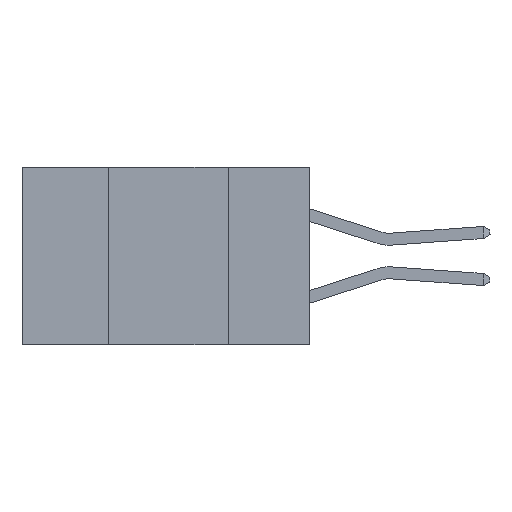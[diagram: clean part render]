
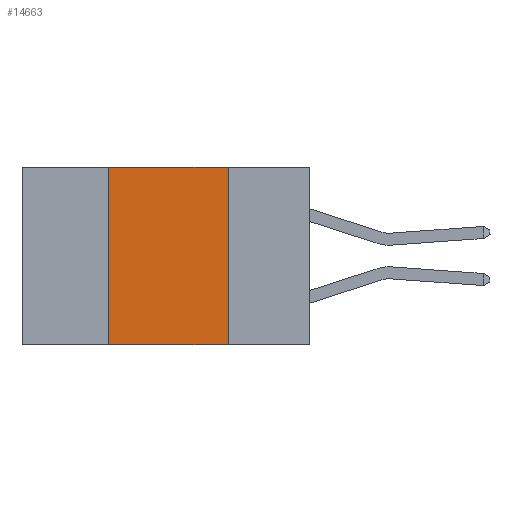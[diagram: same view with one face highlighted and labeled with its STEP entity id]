
A CAD part, left-side view. The second image highlights one B-rep face of the part: STEP entity #14663.
In plain terms, the highlighted planar face has unit normal (-1, 0, 0).
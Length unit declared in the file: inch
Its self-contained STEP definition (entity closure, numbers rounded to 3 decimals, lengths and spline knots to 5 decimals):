
#115 = VECTOR ( 'NONE', #1934, 39.37008 ) ;
#391 = VECTOR ( 'NONE', #13721, 39.37008 ) ;
#867 = CARTESIAN_POINT ( 'NONE',  ( 0., 0.17, 0. ) ) ;
#895 = CARTESIAN_POINT ( 'NONE',  ( 0., 0.42, 0. ) ) ;
#1287 = VERTEX_POINT ( 'NONE', #895 ) ;
#1870 = ORIENTED_EDGE ( 'NONE', *, *, #15285, .F. ) ;
#1934 = DIRECTION ( 'NONE',  ( 0., -1., 0. ) ) ;
#1958 = DIRECTION ( 'NONE',  ( 0., 0., 1. ) ) ;
#2017 = CARTESIAN_POINT ( 'NONE',  ( 0., 0.42, -0.37 ) ) ;
#2029 = CARTESIAN_POINT ( 'NONE',  ( 0., 0.6, 0. ) ) ;
#2528 = FACE_OUTER_BOUND ( 'NONE', #8759, .T. ) ;
#2545 = CARTESIAN_POINT ( 'NONE',  ( 0., 0.17, -0.37 ) ) ;
#2970 = LINE ( 'NONE', #13739, #391 ) ;
#2986 = EDGE_CURVE ( 'NONE', #15452, #8666, #16070, .T. ) ;
#3639 = VECTOR ( 'NONE', #1958, 39.37008 ) ;
#4056 = LINE ( 'NONE', #2017, #3639 ) ;
#4967 = ORIENTED_EDGE ( 'NONE', *, *, #8076, .F. ) ;
#5984 = ORIENTED_EDGE ( 'NONE', *, *, #10369, .T. ) ;
#6494 = DIRECTION ( 'NONE',  ( 0., 0., -1. ) ) ;
#6498 = DIRECTION ( 'NONE',  ( 1., 0., 0. ) ) ;
#6541 = PLANE ( 'NONE',  #10544 ) ;
#6700 = CARTESIAN_POINT ( 'NONE',  ( 0., 0.6, 0. ) ) ;
#7543 = CARTESIAN_POINT ( 'NONE',  ( 0., 0.42, -0.37 ) ) ;
#7635 = VERTEX_POINT ( 'NONE', #7543 ) ;
#8076 = EDGE_CURVE ( 'NONE', #7635, #1287, #4056, .T. ) ;
#8666 = VERTEX_POINT ( 'NONE', #2545 ) ;
#8759 = EDGE_LOOP ( 'NONE', ( #9579, #1870, #4967, #5984 ) ) ;
#9474 = VECTOR ( 'NONE', #13913, 39.37008 ) ;
#9579 = ORIENTED_EDGE ( 'NONE', *, *, #2986, .F. ) ;
#10369 = EDGE_CURVE ( 'NONE', #7635, #8666, #2970, .T. ) ;
#10544 = AXIS2_PLACEMENT_3D ( 'NONE', #6700, #6498, #6494 ) ;
#13208 = LINE ( 'NONE', #2029, #115 ) ;
#13721 = DIRECTION ( 'NONE',  ( 0., -1., 0. ) ) ;
#13739 = CARTESIAN_POINT ( 'NONE',  ( 0., 0.6, -0.37 ) ) ;
#13913 = DIRECTION ( 'NONE',  ( 0., 0., -1. ) ) ;
#13985 = CARTESIAN_POINT ( 'NONE',  ( 0., 0.17, -0.37 ) ) ;
#14663 = ADVANCED_FACE ( 'NONE', ( #2528 ), #6541, .F. ) ;
#15285 = EDGE_CURVE ( 'NONE', #1287, #15452, #13208, .T. ) ;
#15452 = VERTEX_POINT ( 'NONE', #867 ) ;
#16070 = LINE ( 'NONE', #13985, #9474 ) ;
